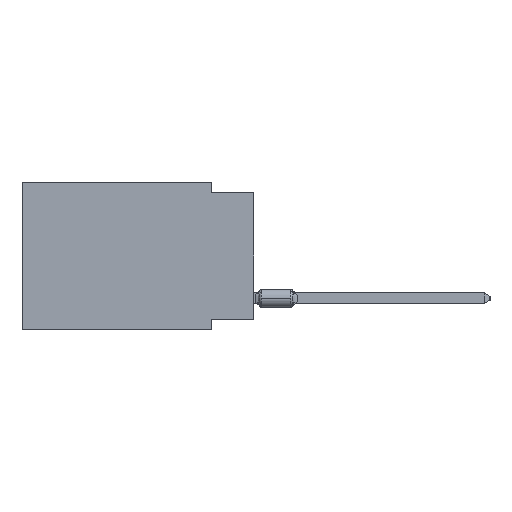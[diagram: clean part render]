
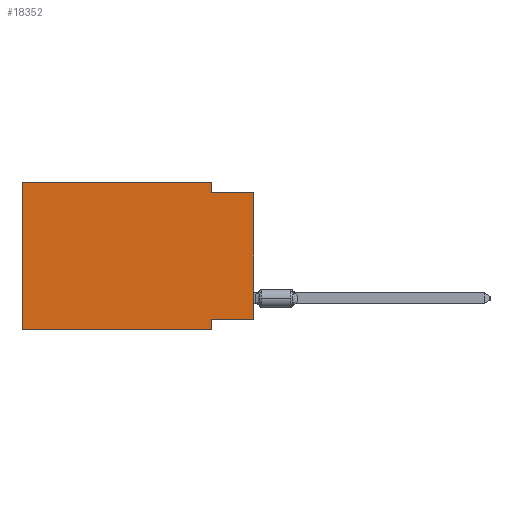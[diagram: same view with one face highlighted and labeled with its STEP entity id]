
A CAD part, left-side view. The second image highlights one B-rep face of the part: STEP entity #18352.
In plain terms, the highlighted planar face has unit normal (-1, 0, 0).
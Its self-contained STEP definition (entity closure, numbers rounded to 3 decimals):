
#1243 = EDGE_CURVE ( 'NONE', #104731, #7610, #107690, .T. ) ;
#2091 = CARTESIAN_POINT ( 'NONE',  ( 0., 2.54, -8.89 ) ) ;
#2572 = EDGE_CURVE ( 'NONE', #7610, #77007, #84317, .T. ) ;
#4968 = CARTESIAN_POINT ( 'NONE',  ( 0., 13.97, -8.89 ) ) ;
#5106 = EDGE_CURVE ( 'NONE', #104731, #49934, #59966, .T. ) ;
#5364 = CARTESIAN_POINT ( 'NONE',  ( 0., 0., -8.255 ) ) ;
#6352 = ORIENTED_EDGE ( 'NONE', *, *, #106205, .F. ) ;
#7610 = VERTEX_POINT ( 'NONE', #92086 ) ;
#8085 = VECTOR ( 'NONE', #60637, 1000. ) ;
#8485 = VECTOR ( 'NONE', #19263, 1000. ) ;
#11442 = EDGE_CURVE ( 'NONE', #46272, #49934, #79895, .T. ) ;
#13019 = CARTESIAN_POINT ( 'NONE',  ( 0., 13.97, 0. ) ) ;
#14089 = VERTEX_POINT ( 'NONE', #72667 ) ;
#15352 = CARTESIAN_POINT ( 'NONE',  ( 0., 13.97, 0. ) ) ;
#15547 = CARTESIAN_POINT ( 'NONE',  ( 0., 2.54, 0. ) ) ;
#18352 = ADVANCED_FACE ( 'NONE', ( #106416 ), #63596, .F. ) ;
#19263 = DIRECTION ( 'NONE',  ( 0., -1., 0. ) ) ;
#21328 = DIRECTION ( 'NONE',  ( 0., 1., 0. ) ) ;
#21599 = VECTOR ( 'NONE', #49979, 1000. ) ;
#22886 = DIRECTION ( 'NONE',  ( 1., 0., 0. ) ) ;
#26042 = CARTESIAN_POINT ( 'NONE',  ( 0., 13.97, 0. ) ) ;
#31518 = EDGE_CURVE ( 'NONE', #108032, #46272, #46616, .T. ) ;
#35632 = CARTESIAN_POINT ( 'NONE',  ( 0., 2.54, -8.255 ) ) ;
#37033 = DIRECTION ( 'NONE',  ( 0., 0., -1. ) ) ;
#37322 = VECTOR ( 'NONE', #91060, 1000. ) ;
#39915 = CARTESIAN_POINT ( 'NONE',  ( 0., 0., -8.255 ) ) ;
#41320 = VECTOR ( 'NONE', #37033, 1000. ) ;
#43656 = AXIS2_PLACEMENT_3D ( 'NONE', #13019, #22886, #48166 ) ;
#45043 = LINE ( 'NONE', #62621, #107370 ) ;
#45891 = ORIENTED_EDGE ( 'NONE', *, *, #79194, .T. ) ;
#46272 = VERTEX_POINT ( 'NONE', #35632 ) ;
#46616 = LINE ( 'NONE', #5364, #55142 ) ;
#47447 = DIRECTION ( 'NONE',  ( 0., 0., 1. ) ) ;
#48166 = DIRECTION ( 'NONE',  ( 0., 0., -1. ) ) ;
#48524 = LINE ( 'NONE', #57324, #96045 ) ;
#48842 = ORIENTED_EDGE ( 'NONE', *, *, #5106, .T. ) ;
#49934 = VERTEX_POINT ( 'NONE', #2091 ) ;
#49979 = DIRECTION ( 'NONE',  ( 0., 0., 1. ) ) ;
#50105 = EDGE_CURVE ( 'NONE', #14089, #77884, #107524, .T. ) ;
#55142 = VECTOR ( 'NONE', #21328, 1000. ) ;
#57324 = CARTESIAN_POINT ( 'NONE',  ( 0., 0., 0. ) ) ;
#58052 = EDGE_LOOP ( 'NONE', ( #45891, #84320, #6352, #82468, #98658, #48842, #76263, #83992 ) ) ;
#59966 = LINE ( 'NONE', #103346, #8485 ) ;
#60637 = DIRECTION ( 'NONE',  ( 0., -1., 0. ) ) ;
#62621 = CARTESIAN_POINT ( 'NONE',  ( 0., 2.54, 0. ) ) ;
#63596 = PLANE ( 'NONE',  #43656 ) ;
#66581 = CARTESIAN_POINT ( 'NONE',  ( 0., 0., -0.635 ) ) ;
#71116 = CARTESIAN_POINT ( 'NONE',  ( 0., 2.54, -8.89 ) ) ;
#72667 = CARTESIAN_POINT ( 'NONE',  ( 0., 2.54, -0.635 ) ) ;
#76263 = ORIENTED_EDGE ( 'NONE', *, *, #11442, .F. ) ;
#77007 = VERTEX_POINT ( 'NONE', #15547 ) ;
#77884 = VERTEX_POINT ( 'NONE', #66581 ) ;
#78589 = DIRECTION ( 'NONE',  ( 0., 0., -1. ) ) ;
#79194 = EDGE_CURVE ( 'NONE', #108032, #77884, #48524, .T. ) ;
#79895 = LINE ( 'NONE', #71116, #41320 ) ;
#82468 = ORIENTED_EDGE ( 'NONE', *, *, #2572, .F. ) ;
#83992 = ORIENTED_EDGE ( 'NONE', *, *, #31518, .F. ) ;
#84317 = LINE ( 'NONE', #26042, #8085 ) ;
#84320 = ORIENTED_EDGE ( 'NONE', *, *, #50105, .F. ) ;
#90509 = CARTESIAN_POINT ( 'NONE',  ( 0., 0., -0.635 ) ) ;
#91060 = DIRECTION ( 'NONE',  ( 0., -1., 0. ) ) ;
#92086 = CARTESIAN_POINT ( 'NONE',  ( 0., 13.97, 0. ) ) ;
#96045 = VECTOR ( 'NONE', #47447, 1000. ) ;
#98658 = ORIENTED_EDGE ( 'NONE', *, *, #1243, .F. ) ;
#103346 = CARTESIAN_POINT ( 'NONE',  ( 0., 13.97, -8.89 ) ) ;
#104731 = VERTEX_POINT ( 'NONE', #4968 ) ;
#106205 = EDGE_CURVE ( 'NONE', #77007, #14089, #45043, .T. ) ;
#106416 = FACE_OUTER_BOUND ( 'NONE', #58052, .T. ) ;
#107370 = VECTOR ( 'NONE', #78589, 1000. ) ;
#107524 = LINE ( 'NONE', #90509, #37322 ) ;
#107690 = LINE ( 'NONE', #15352, #21599 ) ;
#108032 = VERTEX_POINT ( 'NONE', #39915 ) ;
